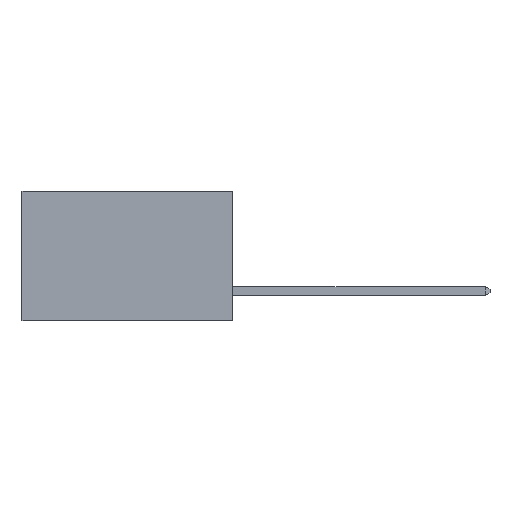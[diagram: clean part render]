
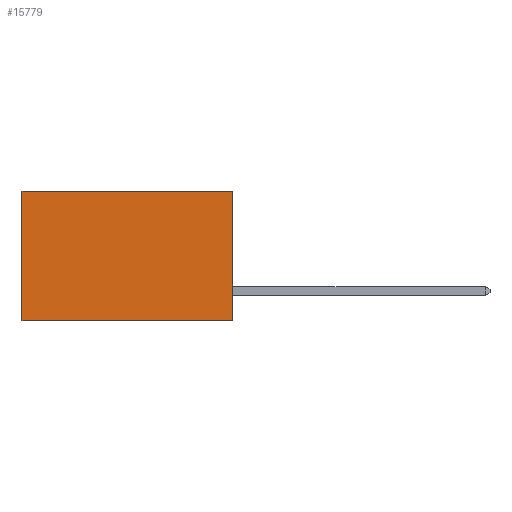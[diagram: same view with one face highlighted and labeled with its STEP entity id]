
A CAD part, left-side view. The second image highlights one B-rep face of the part: STEP entity #15779.
In plain terms, the highlighted planar face has unit normal (-1, 0, 0).
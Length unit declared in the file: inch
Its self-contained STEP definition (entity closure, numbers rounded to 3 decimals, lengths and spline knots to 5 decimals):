
#21 = EDGE_LOOP ( 'NONE', ( #2558, #9907, #15408, #5228 ) ) ;
#44 = DIRECTION ( 'NONE',  ( 0., 0., -1. ) ) ;
#56 = VECTOR ( 'NONE', #473, 39.37008 ) ;
#473 = DIRECTION ( 'NONE',  ( 0., 0., -1. ) ) ;
#1143 = EDGE_CURVE ( 'NONE', #7557, #6151, #2771, .T. ) ;
#1754 = DIRECTION ( 'NONE',  ( 0., 1., 0. ) ) ;
#2204 = CARTESIAN_POINT ( 'NONE',  ( 0.2875, 0., -0.37 ) ) ;
#2548 = CARTESIAN_POINT ( 'NONE',  ( 0.2875, 0.6, 0. ) ) ;
#2558 = ORIENTED_EDGE ( 'NONE', *, *, #13076, .T. ) ;
#2771 = LINE ( 'NONE', #2204, #15733 ) ;
#4756 = DIRECTION ( 'NONE',  ( 0., 1., 0. ) ) ;
#4757 = CARTESIAN_POINT ( 'NONE',  ( 0.2875, 0.6, -0.37 ) ) ;
#5144 = VERTEX_POINT ( 'NONE', #11712 ) ;
#5176 = CARTESIAN_POINT ( 'NONE',  ( 0.2875, 0., 0. ) ) ;
#5228 = ORIENTED_EDGE ( 'NONE', *, *, #9485, .T. ) ;
#5706 = EDGE_CURVE ( 'NONE', #5144, #7557, #6005, .T. ) ;
#6005 = LINE ( 'NONE', #11326, #9025 ) ;
#6151 = VERTEX_POINT ( 'NONE', #4757 ) ;
#7312 = CARTESIAN_POINT ( 'NONE',  ( 0.2875, 0., 0. ) ) ;
#7557 = VERTEX_POINT ( 'NONE', #12213 ) ;
#7747 = DIRECTION ( 'NONE',  ( 1., 0., 0. ) ) ;
#8437 = FACE_OUTER_BOUND ( 'NONE', #21, .T. ) ;
#8485 = LINE ( 'NONE', #7312, #11845 ) ;
#9025 = VECTOR ( 'NONE', #10222, 39.37008 ) ;
#9485 = EDGE_CURVE ( 'NONE', #5144, #15242, #8485, .T. ) ;
#9907 = ORIENTED_EDGE ( 'NONE', *, *, #1143, .F. ) ;
#10222 = DIRECTION ( 'NONE',  ( 0., 0., -1. ) ) ;
#11030 = AXIS2_PLACEMENT_3D ( 'NONE', #5176, #7747, #44 ) ;
#11326 = CARTESIAN_POINT ( 'NONE',  ( 0.2875, 0., 0. ) ) ;
#11525 = PLANE ( 'NONE',  #11030 ) ;
#11712 = CARTESIAN_POINT ( 'NONE',  ( 0.2875, 0., 0. ) ) ;
#11845 = VECTOR ( 'NONE', #4756, 39.37008 ) ;
#12213 = CARTESIAN_POINT ( 'NONE',  ( 0.2875, 0., -0.37 ) ) ;
#13076 = EDGE_CURVE ( 'NONE', #15242, #6151, #14715, .T. ) ;
#14715 = LINE ( 'NONE', #15567, #56 ) ;
#15242 = VERTEX_POINT ( 'NONE', #2548 ) ;
#15408 = ORIENTED_EDGE ( 'NONE', *, *, #5706, .F. ) ;
#15567 = CARTESIAN_POINT ( 'NONE',  ( 0.2875, 0.6, 0. ) ) ;
#15733 = VECTOR ( 'NONE', #1754, 39.37008 ) ;
#15779 = ADVANCED_FACE ( 'NONE', ( #8437 ), #11525, .F. ) ;
